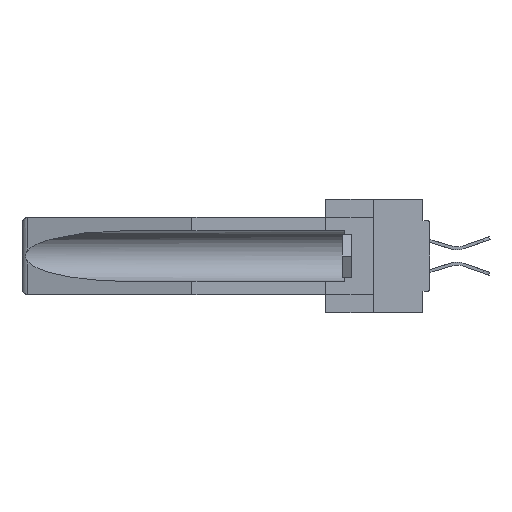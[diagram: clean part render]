
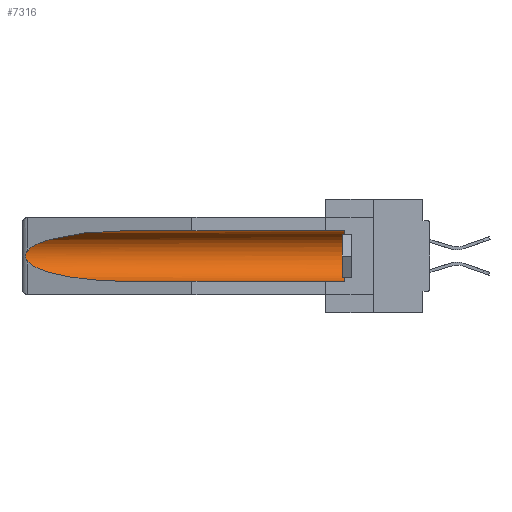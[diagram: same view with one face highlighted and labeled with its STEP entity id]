
A CAD part, left-side view. The second image highlights one B-rep face of the part: STEP entity #7316.
In plain terms, the highlighted cylindrical face has radius 2.857 mm (diameter 5.715 mm), a partial arc.
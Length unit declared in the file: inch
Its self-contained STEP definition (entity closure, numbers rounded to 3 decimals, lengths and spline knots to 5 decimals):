
#875 = CARTESIAN_POINT ( 'NONE',  ( 0.155, -0.30754, -0.059 ) ) ;
#966 = EDGE_CURVE ( 'NONE', #10698, #26057, #31150, .T. ) ;
#2097 = VERTEX_POINT ( 'NONE', #13865 ) ;
#2665 = ORIENTED_EDGE ( 'NONE', *, *, #29430, .T. ) ;
#2862 = ORIENTED_EDGE ( 'NONE', *, *, #8906, .T. ) ;
#3468 = DIRECTION ( 'NONE',  ( 0., 0., 1. ) ) ;
#4543 = VERTEX_POINT ( 'NONE', #22290 ) ;
#6862 = CARTESIAN_POINT ( 'NONE',  ( 0.2673, 1.5327, -0.16383 ) ) ;
#7316 = ADVANCED_FACE ( 'NONE', ( #23983 ), #24805, .F. ) ;
#7616 = ORIENTED_EDGE ( 'NONE', *, *, #34983, .T. ) ;
#7761 = DIRECTION ( 'NONE',  ( 0., -1., 0. ) ) ;
#7845 = VECTOR ( 'NONE', #8651, 39.37008 ) ;
#8637 = CIRCLE ( 'NONE', #28693, 0.1125 ) ;
#8651 = DIRECTION ( 'NONE',  ( 0., 1., 0. ) ) ;
#8906 = EDGE_CURVE ( 'NONE', #33541, #4543, #10242, .T. ) ;
#9169 = CARTESIAN_POINT ( 'NONE',  ( 0.155, 1.07973, -0.059 ) ) ;
#9575 = CARTESIAN_POINT ( 'NONE',  ( 0.2673, 1.53269, -0.17917 ) ) ;
#10242 = LINE ( 'NONE', #875, #11466 ) ;
#10698 = VERTEX_POINT ( 'NONE', #24944 ) ;
#11087 =( BOUNDED_CURVE ( )  B_SPLINE_CURVE ( 3, ( #9169, #17113, #22898, #14727 ),
 .UNSPECIFIED., .F., .F. ) 
 B_SPLINE_CURVE_WITH_KNOTS ( ( 4, 4 ),
 ( 4.71239, 6.08839 ),
 .UNSPECIFIED. ) 
 CURVE ( )  GEOMETRIC_REPRESENTATION_ITEM ( )  RATIONAL_B_SPLINE_CURVE ( ( 1., 0.848, 0.848, 1. ) ) 
 REPRESENTATION_ITEM ( '' )  );
#11466 = VECTOR ( 'NONE', #19387, 39.37008 ) ;
#11684 = CARTESIAN_POINT ( 'NONE',  ( 0.26537, 1.52718, -0.19328 ) ) ;
#11704 = B_SPLINE_CURVE_WITH_KNOTS ( 'NONE', 3,
 ( #26027, #23298, #33865, #6862, #34095, #25784, #9575, #28517, #33984, #17771 ),
 .UNSPECIFIED., .F., .F.,
 ( 4, 2, 2, 2, 4 ),
 ( 0., 0.00029, 0.00058, 0.00087, 0.00117 ),
 .UNSPECIFIED. ) ;
#13865 = CARTESIAN_POINT ( 'NONE',  ( 0.26537, 1.52718, -0.14972 ) ) ;
#14005 = VERTEX_POINT ( 'NONE', #11684 ) ;
#14727 = CARTESIAN_POINT ( 'NONE',  ( 0.26537, 1.52718, -0.14972 ) ) ;
#16921 =( BOUNDED_CURVE ( )  B_SPLINE_CURVE ( 3, ( #29395, #32140, #34846, #26923 ),
 .UNSPECIFIED., .F., .T. ) 
 B_SPLINE_CURVE_WITH_KNOTS ( ( 4, 4 ),
 ( 0.1948, 1.5708 ),
 .UNSPECIFIED. ) 
 CURVE ( )  GEOMETRIC_REPRESENTATION_ITEM ( )  RATIONAL_B_SPLINE_CURVE ( ( 1., 0.848, 0.848, 1. ) ) 
 REPRESENTATION_ITEM ( '' )  );
#17113 = CARTESIAN_POINT ( 'NONE',  ( 0.21114, 1.30732, -0.059 ) ) ;
#17771 = CARTESIAN_POINT ( 'NONE',  ( 0.26537, 1.52718, -0.19328 ) ) ;
#18114 = CARTESIAN_POINT ( 'NONE',  ( 0.155, 0.126, -0.1715 ) ) ;
#19387 = DIRECTION ( 'NONE',  ( 0., 1., 0. ) ) ;
#19409 = EDGE_LOOP ( 'NONE', ( #7616, #25514, #23788, #21404, #2665, #2862 ) ) ;
#19786 = EDGE_CURVE ( 'NONE', #2097, #14005, #11704, .T. ) ;
#19846 = DIRECTION ( 'NONE',  ( 0., 1., 0. ) ) ;
#21404 = ORIENTED_EDGE ( 'NONE', *, *, #966, .F. ) ;
#22290 = CARTESIAN_POINT ( 'NONE',  ( 0.155, 1.07973, -0.059 ) ) ;
#22898 = CARTESIAN_POINT ( 'NONE',  ( 0.25451, 1.48313, -0.09465 ) ) ;
#23177 = CARTESIAN_POINT ( 'NONE',  ( 0.155, 0.126, -0.059 ) ) ;
#23298 = CARTESIAN_POINT ( 'NONE',  ( 0.26597, 1.52961, -0.15275 ) ) ;
#23788 = ORIENTED_EDGE ( 'NONE', *, *, #29772, .T. ) ;
#23983 = FACE_OUTER_BOUND ( 'NONE', #19409, .T. ) ;
#24805 = CYLINDRICAL_SURFACE ( 'NONE', #27948, 0.1125 ) ;
#24944 = CARTESIAN_POINT ( 'NONE',  ( 0.155, 0.126, -0.284 ) ) ;
#25514 = ORIENTED_EDGE ( 'NONE', *, *, #19786, .T. ) ;
#25784 = CARTESIAN_POINT ( 'NONE',  ( 0.2675, 1.53308, -0.17534 ) ) ;
#26027 = CARTESIAN_POINT ( 'NONE',  ( 0.26537, 1.52718, -0.14972 ) ) ;
#26057 = VERTEX_POINT ( 'NONE', #26908 ) ;
#26908 = CARTESIAN_POINT ( 'NONE',  ( 0.155, 1.07973, -0.284 ) ) ;
#26923 = CARTESIAN_POINT ( 'NONE',  ( 0.155, 1.07973, -0.284 ) ) ;
#27366 = CARTESIAN_POINT ( 'NONE',  ( 0.155, -0.30754, -0.284 ) ) ;
#27948 = AXIS2_PLACEMENT_3D ( 'NONE', #33575, #19846, #3468 ) ;
#28517 = CARTESIAN_POINT ( 'NONE',  ( 0.26655, 1.53094, -0.18657 ) ) ;
#28693 = AXIS2_PLACEMENT_3D ( 'NONE', #18114, #7761, #32185 ) ;
#29395 = CARTESIAN_POINT ( 'NONE',  ( 0.26537, 1.52718, -0.19328 ) ) ;
#29430 = EDGE_CURVE ( 'NONE', #10698, #33541, #8637, .T. ) ;
#29772 = EDGE_CURVE ( 'NONE', #14005, #26057, #16921, .T. ) ;
#31150 = LINE ( 'NONE', #27366, #7845 ) ;
#32140 = CARTESIAN_POINT ( 'NONE',  ( 0.25451, 1.48313, -0.24835 ) ) ;
#32185 = DIRECTION ( 'NONE',  ( 0., 0., 1. ) ) ;
#33541 = VERTEX_POINT ( 'NONE', #23177 ) ;
#33575 = CARTESIAN_POINT ( 'NONE',  ( 0.155, -0.30754, -0.1715 ) ) ;
#33865 = CARTESIAN_POINT ( 'NONE',  ( 0.26654, 1.53092, -0.15636 ) ) ;
#33984 = CARTESIAN_POINT ( 'NONE',  ( 0.26597, 1.5296, -0.19026 ) ) ;
#34095 = CARTESIAN_POINT ( 'NONE',  ( 0.2675, 1.53308, -0.16763 ) ) ;
#34846 = CARTESIAN_POINT ( 'NONE',  ( 0.21114, 1.30732, -0.284 ) ) ;
#34983 = EDGE_CURVE ( 'NONE', #4543, #2097, #11087, .T. ) ;
